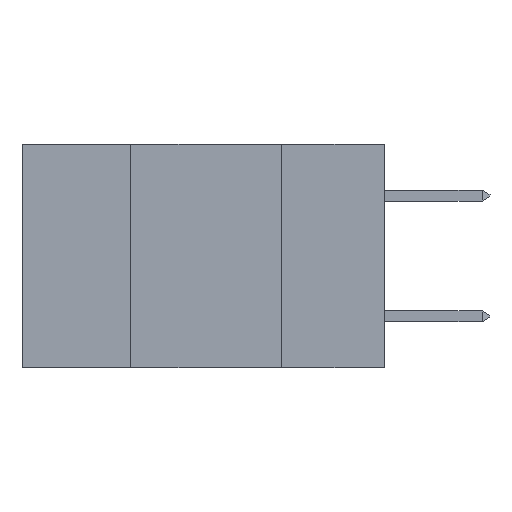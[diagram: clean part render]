
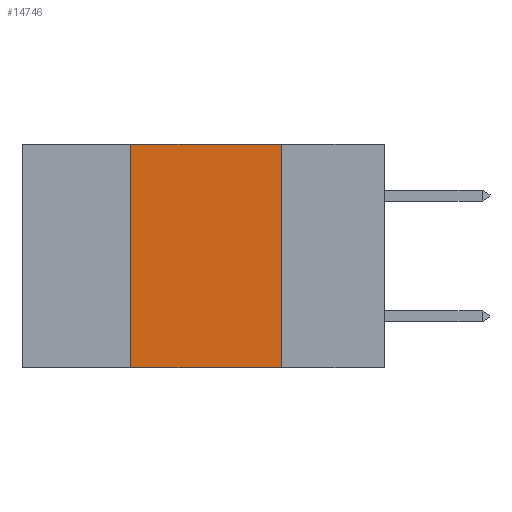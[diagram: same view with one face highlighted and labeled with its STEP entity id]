
A CAD part, left-side view. The second image highlights one B-rep face of the part: STEP entity #14746.
In plain terms, the highlighted planar face has unit normal (-1, 0, 0).
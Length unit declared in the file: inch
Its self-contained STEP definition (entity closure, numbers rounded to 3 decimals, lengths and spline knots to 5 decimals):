
#8 = CARTESIAN_POINT ( 'NONE',  ( 0., 0.6, 0. ) ) ;
#389 = CARTESIAN_POINT ( 'NONE',  ( 0., 0.17, -0.37 ) ) ;
#570 = DIRECTION ( 'NONE',  ( 0., -1., 0. ) ) ;
#2824 = VECTOR ( 'NONE', #9566, 39.37008 ) ;
#2893 = EDGE_CURVE ( 'NONE', #9532, #13967, #6077, .T. ) ;
#3462 = VECTOR ( 'NONE', #11511, 39.37008 ) ;
#3586 = CARTESIAN_POINT ( 'NONE',  ( 0., 0.17, 0. ) ) ;
#3677 = VECTOR ( 'NONE', #570, 39.37008 ) ;
#3736 = CARTESIAN_POINT ( 'NONE',  ( 0., 0.42, -0.37 ) ) ;
#4216 = EDGE_CURVE ( 'NONE', #11903, #4236, #4302, .T. ) ;
#4236 = VERTEX_POINT ( 'NONE', #6300 ) ;
#4302 = LINE ( 'NONE', #9583, #7106 ) ;
#5121 = DIRECTION ( 'NONE',  ( 0., 0., -1. ) ) ;
#5919 = EDGE_CURVE ( 'NONE', #4236, #9532, #9634, .T. ) ;
#6077 = LINE ( 'NONE', #3586, #2824 ) ;
#6300 = CARTESIAN_POINT ( 'NONE',  ( 0., 0.42, 0. ) ) ;
#6519 = EDGE_CURVE ( 'NONE', #11903, #13967, #6660, .T. ) ;
#6595 = ORIENTED_EDGE ( 'NONE', *, *, #2893, .F. ) ;
#6660 = LINE ( 'NONE', #7976, #3462 ) ;
#7106 = VECTOR ( 'NONE', #11875, 39.37008 ) ;
#7890 = CARTESIAN_POINT ( 'NONE',  ( 0., 0.6, 0. ) ) ;
#7976 = CARTESIAN_POINT ( 'NONE',  ( 0., 0.6, -0.37 ) ) ;
#8058 = ORIENTED_EDGE ( 'NONE', *, *, #4216, .F. ) ;
#8612 = PLANE ( 'NONE',  #14143 ) ;
#9532 = VERTEX_POINT ( 'NONE', #15322 ) ;
#9566 = DIRECTION ( 'NONE',  ( 0., 0., -1. ) ) ;
#9583 = CARTESIAN_POINT ( 'NONE',  ( 0., 0.42, 0. ) ) ;
#9634 = LINE ( 'NONE', #7890, #3677 ) ;
#11511 = DIRECTION ( 'NONE',  ( 0., -1., 0. ) ) ;
#11875 = DIRECTION ( 'NONE',  ( 0., 0., 1. ) ) ;
#11903 = VERTEX_POINT ( 'NONE', #3736 ) ;
#12135 = DIRECTION ( 'NONE',  ( 1., 0., 0. ) ) ;
#12214 = EDGE_LOOP ( 'NONE', ( #6595, #13890, #8058, #14615 ) ) ;
#12463 = FACE_OUTER_BOUND ( 'NONE', #12214, .T. ) ;
#13890 = ORIENTED_EDGE ( 'NONE', *, *, #5919, .F. ) ;
#13967 = VERTEX_POINT ( 'NONE', #389 ) ;
#14143 = AXIS2_PLACEMENT_3D ( 'NONE', #8, #12135, #5121 ) ;
#14615 = ORIENTED_EDGE ( 'NONE', *, *, #6519, .T. ) ;
#14746 = ADVANCED_FACE ( 'NONE', ( #12463 ), #8612, .F. ) ;
#15322 = CARTESIAN_POINT ( 'NONE',  ( 0., 0.17, 0. ) ) ;
